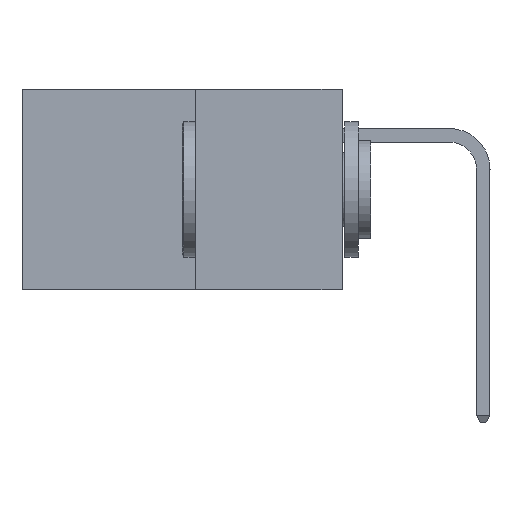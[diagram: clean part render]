
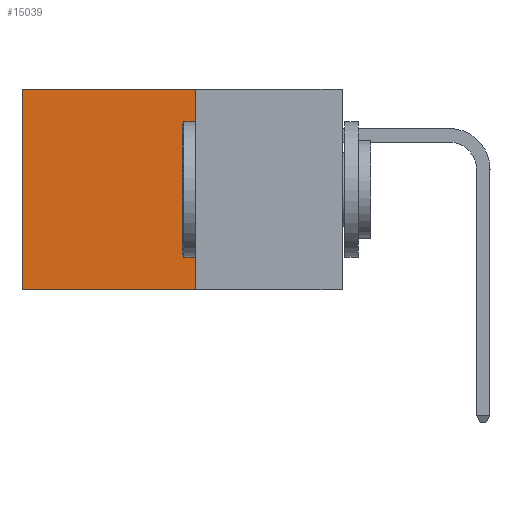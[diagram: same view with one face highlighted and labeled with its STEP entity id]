
A CAD part, left-side view. The second image highlights one B-rep face of the part: STEP entity #15039.
In plain terms, the highlighted planar face has unit normal (-1, 0, 0).
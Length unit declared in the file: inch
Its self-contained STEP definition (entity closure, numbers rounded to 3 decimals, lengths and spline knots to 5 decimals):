
#93 = ORIENTED_EDGE ( 'NONE', *, *, #7885, .T. ) ;
#107 = EDGE_CURVE ( 'NONE', #2485, #3390, #4145, .T. ) ;
#460 = VECTOR ( 'NONE', #4251, 39.37008 ) ;
#520 = CARTESIAN_POINT ( 'NONE',  ( 0.277, 0.27, 0. ) ) ;
#961 = LINE ( 'NONE', #16086, #5045 ) ;
#1065 = DIRECTION ( 'NONE',  ( 0., 0., -1. ) ) ;
#1076 = DIRECTION ( 'NONE',  ( 0., 1., 0. ) ) ;
#1736 = AXIS2_PLACEMENT_3D ( 'NONE', #6524, #9244, #1065 ) ;
#2104 = CARTESIAN_POINT ( 'NONE',  ( 0.277, 0.27, -0.37 ) ) ;
#2485 = VERTEX_POINT ( 'NONE', #2104 ) ;
#3390 = VERTEX_POINT ( 'NONE', #16381 ) ;
#4145 = LINE ( 'NONE', #14346, #460 ) ;
#4251 = DIRECTION ( 'NONE',  ( 0., 1., 0. ) ) ;
#5045 = VECTOR ( 'NONE', #14780, 39.37008 ) ;
#5218 = CARTESIAN_POINT ( 'NONE',  ( 0.277, 0.27, 0. ) ) ;
#5774 = CARTESIAN_POINT ( 'NONE',  ( 0.277, 0.27, -0.37 ) ) ;
#6524 = CARTESIAN_POINT ( 'NONE',  ( 0.277, 0.27, -0.37 ) ) ;
#6688 = FACE_OUTER_BOUND ( 'NONE', #8041, .T. ) ;
#7691 = VECTOR ( 'NONE', #13596, 39.37008 ) ;
#7885 = EDGE_CURVE ( 'NONE', #16850, #13709, #15933, .T. ) ;
#8041 = EDGE_LOOP ( 'NONE', ( #15954, #10686, #14725, #93 ) ) ;
#9244 = DIRECTION ( 'NONE',  ( 1., 0., 0. ) ) ;
#10686 = ORIENTED_EDGE ( 'NONE', *, *, #107, .F. ) ;
#11185 = LINE ( 'NONE', #5774, #7691 ) ;
#11693 = CARTESIAN_POINT ( 'NONE',  ( 0.277, 0.59, 0. ) ) ;
#11752 = VECTOR ( 'NONE', #1076, 39.37008 ) ;
#13498 = EDGE_CURVE ( 'NONE', #13709, #3390, #961, .T. ) ;
#13596 = DIRECTION ( 'NONE',  ( 0., 0., -1. ) ) ;
#13709 = VERTEX_POINT ( 'NONE', #11693 ) ;
#14346 = CARTESIAN_POINT ( 'NONE',  ( 0.277, 0.27, -0.37 ) ) ;
#14725 = ORIENTED_EDGE ( 'NONE', *, *, #16073, .F. ) ;
#14780 = DIRECTION ( 'NONE',  ( 0., 0., -1. ) ) ;
#15039 = ADVANCED_FACE ( 'NONE', ( #6688 ), #16826, .F. ) ;
#15933 = LINE ( 'NONE', #5218, #11752 ) ;
#15954 = ORIENTED_EDGE ( 'NONE', *, *, #13498, .T. ) ;
#16073 = EDGE_CURVE ( 'NONE', #16850, #2485, #11185, .T. ) ;
#16086 = CARTESIAN_POINT ( 'NONE',  ( 0.277, 0.59, -0.37 ) ) ;
#16381 = CARTESIAN_POINT ( 'NONE',  ( 0.277, 0.59, -0.37 ) ) ;
#16826 = PLANE ( 'NONE',  #1736 ) ;
#16850 = VERTEX_POINT ( 'NONE', #520 ) ;
